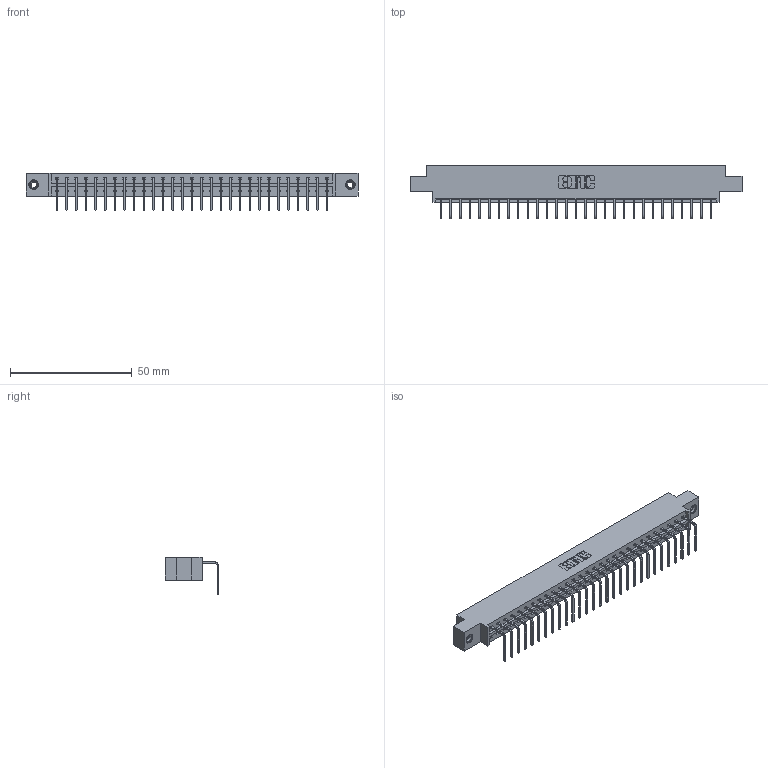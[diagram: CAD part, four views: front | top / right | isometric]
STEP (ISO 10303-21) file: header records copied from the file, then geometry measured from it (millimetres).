
FILE_DESCRIPTION (( 'STEP AP203' ), '1' );
FILE_NAME ('833-029-558-608.STEP', '2020-06-02T11:30:21', ( '' ), ( '' ), 'SwSTEP 2.0', 'SolidWorks 2020', '' );
FILE_SCHEMA (( 'CONFIG_CONTROL_DESIGN' ));
Length unit declared in the file: inch
Products named in the file (4): 345-292-001_558 Tail - 2; 833 Part_Offset - .156 Dia - TI; 345-250-001_345-250-003-102; 833-029-558-608
Assembly tree (32 placements, depth 2):
  833-029-558-608
    833 Part_Offset - .156 Dia - TI
    345-292-001_558 Tail - 2  x29
    345-250-001_345-250-003-102  x2
Bounding box: 136.45 x 22.17 x 15.37 mm (x, y, z)
Volume: 13481.1 mm3; surface area: 15317.6 mm2
Topology: 32 solids, 32 shells, 1918 faces, 5737 edges, 3778 vertices
Faces by surface type: plane 1382, cylinder 520, cone 12, torus 4
Entity records: 20812 total; most frequent: CARTESIAN_POINT 3576, ORIENTED_EDGE 3534, DIRECTION 3075, EDGE_CURVE 1767, LINE 1619, VECTOR 1619, VERTEX_POINT 1172, AXIS2_PLACEMENT_3D 728
